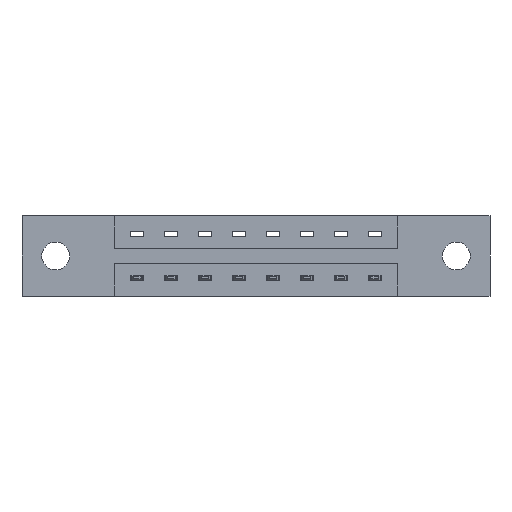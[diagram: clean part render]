
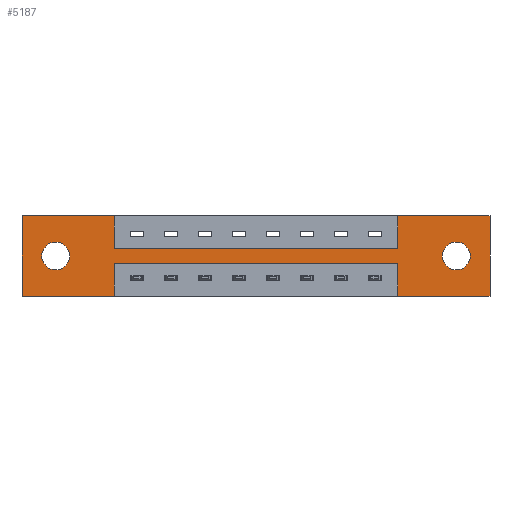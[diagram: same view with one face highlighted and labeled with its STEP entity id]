
A CAD part, front view. The second image highlights one B-rep face of the part: STEP entity #5187.
In plain terms, the highlighted planar face has unit normal (0, -1, 0).
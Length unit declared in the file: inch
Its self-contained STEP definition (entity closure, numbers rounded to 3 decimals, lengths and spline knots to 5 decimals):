
#52 = CARTESIAN_POINT ( 'NONE',  ( 1.729, 0., -0.37 ) ) ;
#64 = ORIENTED_EDGE ( 'NONE', *, *, #7880, .F. ) ;
#75 = CARTESIAN_POINT ( 'NONE',  ( 0.425, 0., -0.37 ) ) ;
#120 = CARTESIAN_POINT ( 'NONE',  ( 0., 0., 0. ) ) ;
#176 = CARTESIAN_POINT ( 'NONE',  ( 1.729, 0., 0. ) ) ;
#195 = LINE ( 'NONE', #4023, #8301 ) ;
#264 = CARTESIAN_POINT ( 'NONE',  ( 0., 0., 0. ) ) ;
#353 = ORIENTED_EDGE ( 'NONE', *, *, #9726, .F. ) ;
#450 = DIRECTION ( 'NONE',  ( 0., 1., 0. ) ) ;
#461 = VERTEX_POINT ( 'NONE', #4950 ) ;
#593 = VERTEX_POINT ( 'NONE', #9999 ) ;
#688 = LINE ( 'NONE', #8613, #2785 ) ;
#726 = EDGE_CURVE ( 'NONE', #593, #8300, #8420, .T. ) ;
#777 = EDGE_LOOP ( 'NONE', ( #1877, #1824 ) ) ;
#804 = CARTESIAN_POINT ( 'NONE',  ( 1.729, 0., -0.37 ) ) ;
#881 = LINE ( 'NONE', #1206, #3832 ) ;
#917 = CARTESIAN_POINT ( 'NONE',  ( 1.999, 0., -0.185 ) ) ;
#940 = VERTEX_POINT ( 'NONE', #6692 ) ;
#950 = DIRECTION ( 'NONE',  ( 0., 0., -1. ) ) ;
#1182 = EDGE_CURVE ( 'NONE', #461, #4940, #195, .T. ) ;
#1206 = CARTESIAN_POINT ( 'NONE',  ( 0., 0., 0. ) ) ;
#1278 = DIRECTION ( 'NONE',  ( 0., 1., 0. ) ) ;
#1452 = CIRCLE ( 'NONE', #3886, 0.064 ) ;
#1652 = LINE ( 'NONE', #5643, #7685 ) ;
#1708 = DIRECTION ( 'NONE',  ( 0., 1., 0. ) ) ;
#1778 = CIRCLE ( 'NONE', #5254, 0.064 ) ;
#1800 = EDGE_CURVE ( 'NONE', #6909, #2891, #7674, .T. ) ;
#1824 = ORIENTED_EDGE ( 'NONE', *, *, #1992, .T. ) ;
#1877 = ORIENTED_EDGE ( 'NONE', *, *, #9441, .T. ) ;
#1889 = DIRECTION ( 'NONE',  ( 0., 0., -1. ) ) ;
#1926 = VERTEX_POINT ( 'NONE', #7543 ) ;
#1992 = EDGE_CURVE ( 'NONE', #8514, #6498, #2105, .T. ) ;
#2105 = CIRCLE ( 'NONE', #4725, 0.064 ) ;
#2249 = DIRECTION ( 'NONE',  ( -1., 0., 0. ) ) ;
#2255 = CARTESIAN_POINT ( 'NONE',  ( 0., 0., -0.37 ) ) ;
#2265 = VECTOR ( 'NONE', #7362, 39.37008 ) ;
#2330 = EDGE_LOOP ( 'NONE', ( #5724, #7403, #7602, #4914, #9261, #9530, #353, #2766, #64, #7367, #5895, #9300 ) ) ;
#2389 = CARTESIAN_POINT ( 'NONE',  ( 0., 0., -0.37 ) ) ;
#2502 = EDGE_CURVE ( 'NONE', #2891, #1926, #881, .T. ) ;
#2766 = ORIENTED_EDGE ( 'NONE', *, *, #1182, .F. ) ;
#2785 = VECTOR ( 'NONE', #7009, 39.37008 ) ;
#2854 = DIRECTION ( 'NONE',  ( 0., 0., 1. ) ) ;
#2891 = VERTEX_POINT ( 'NONE', #120 ) ;
#3141 = CARTESIAN_POINT ( 'NONE',  ( 0.425, 0., -0.22 ) ) ;
#3403 = DIRECTION ( 'NONE',  ( 0., -1., 0. ) ) ;
#3424 = CARTESIAN_POINT ( 'NONE',  ( 0.155, 0., -0.121 ) ) ;
#3506 = PLANE ( 'NONE',  #7086 ) ;
#3513 = ORIENTED_EDGE ( 'NONE', *, *, #4875, .T. ) ;
#3809 = VERTEX_POINT ( 'NONE', #804 ) ;
#3832 = VECTOR ( 'NONE', #5127, 39.37008 ) ;
#3841 = EDGE_LOOP ( 'NONE', ( #3513, #7511 ) ) ;
#3884 = DIRECTION ( 'NONE',  ( 0., 0., -1. ) ) ;
#3886 = AXIS2_PLACEMENT_3D ( 'NONE', #6700, #1278, #5930 ) ;
#4023 = CARTESIAN_POINT ( 'NONE',  ( 0.425, 0., -0.15 ) ) ;
#4321 = CARTESIAN_POINT ( 'NONE',  ( 0., 0., -0.37 ) ) ;
#4501 = CIRCLE ( 'NONE', #9730, 0.064 ) ;
#4725 = AXIS2_PLACEMENT_3D ( 'NONE', #6296, #7839, #10087 ) ;
#4744 = DIRECTION ( 'NONE',  ( 0., 0., 1. ) ) ;
#4875 = EDGE_CURVE ( 'NONE', #940, #8865, #1452, .T. ) ;
#4914 = ORIENTED_EDGE ( 'NONE', *, *, #6810, .F. ) ;
#4940 = VERTEX_POINT ( 'NONE', #9097 ) ;
#4950 = CARTESIAN_POINT ( 'NONE',  ( 0.425, 0., -0.15 ) ) ;
#5127 = DIRECTION ( 'NONE',  ( 1., 0., 0. ) ) ;
#5187 = ADVANCED_FACE ( 'NONE', ( #5380, #8445, #6982 ), #3506, .T. ) ;
#5199 = LINE ( 'NONE', #2389, #8622 ) ;
#5254 = AXIS2_PLACEMENT_3D ( 'NONE', #7581, #450, #2854 ) ;
#5380 = FACE_BOUND ( 'NONE', #3841, .T. ) ;
#5643 = CARTESIAN_POINT ( 'NONE',  ( 1.729, 0., 0. ) ) ;
#5709 = VECTOR ( 'NONE', #6383, 39.37008 ) ;
#5724 = ORIENTED_EDGE ( 'NONE', *, *, #6390, .F. ) ;
#5735 = EDGE_CURVE ( 'NONE', #9885, #6605, #688, .T. ) ;
#5749 = VECTOR ( 'NONE', #8586, 39.37008 ) ;
#5837 = EDGE_CURVE ( 'NONE', #8865, #940, #4501, .T. ) ;
#5895 = ORIENTED_EDGE ( 'NONE', *, *, #1800, .F. ) ;
#5930 = DIRECTION ( 'NONE',  ( 0., 0., -1. ) ) ;
#6005 = DIRECTION ( 'NONE',  ( -1., 0., 0. ) ) ;
#6296 = CARTESIAN_POINT ( 'NONE',  ( 0.155, 0., -0.185 ) ) ;
#6314 = CARTESIAN_POINT ( 'NONE',  ( 0.425, 0., 0. ) ) ;
#6341 = CARTESIAN_POINT ( 'NONE',  ( 0.425, 0., -0.37 ) ) ;
#6383 = DIRECTION ( 'NONE',  ( 0., 0., 1. ) ) ;
#6390 = EDGE_CURVE ( 'NONE', #8300, #7465, #7914, .T. ) ;
#6497 = DIRECTION ( 'NONE',  ( 0., 0., 1. ) ) ;
#6498 = VERTEX_POINT ( 'NONE', #3424 ) ;
#6605 = VERTEX_POINT ( 'NONE', #8431 ) ;
#6692 = CARTESIAN_POINT ( 'NONE',  ( 1.999, 0., -0.121 ) ) ;
#6700 = CARTESIAN_POINT ( 'NONE',  ( 1.999, 0., -0.185 ) ) ;
#6810 = EDGE_CURVE ( 'NONE', #6605, #3809, #9123, .T. ) ;
#6909 = VERTEX_POINT ( 'NONE', #2255 ) ;
#6954 = CARTESIAN_POINT ( 'NONE',  ( 0.425, 0., -0.22 ) ) ;
#6982 = FACE_OUTER_BOUND ( 'NONE', #2330, .T. ) ;
#7009 = DIRECTION ( 'NONE',  ( 0., 0., -1. ) ) ;
#7086 = AXIS2_PLACEMENT_3D ( 'NONE', #4321, #3403, #7387 ) ;
#7155 = DIRECTION ( 'NONE',  ( 1., 0., 0. ) ) ;
#7172 = CARTESIAN_POINT ( 'NONE',  ( 1.999, 0., -0.249 ) ) ;
#7300 = CARTESIAN_POINT ( 'NONE',  ( 2.154, 0., 0. ) ) ;
#7342 = LINE ( 'NONE', #7999, #2265 ) ;
#7362 = DIRECTION ( 'NONE',  ( 1., 0., 0. ) ) ;
#7367 = ORIENTED_EDGE ( 'NONE', *, *, #2502, .F. ) ;
#7387 = DIRECTION ( 'NONE',  ( 0., 0., -1. ) ) ;
#7403 = ORIENTED_EDGE ( 'NONE', *, *, #726, .F. ) ;
#7465 = VERTEX_POINT ( 'NONE', #6341 ) ;
#7471 = EDGE_CURVE ( 'NONE', #3809, #593, #8389, .T. ) ;
#7511 = ORIENTED_EDGE ( 'NONE', *, *, #5837, .T. ) ;
#7543 = CARTESIAN_POINT ( 'NONE',  ( 0.425, 0., 0. ) ) ;
#7563 = VECTOR ( 'NONE', #4744, 39.37008 ) ;
#7577 = VECTOR ( 'NONE', #1889, 39.37008 ) ;
#7581 = CARTESIAN_POINT ( 'NONE',  ( 0.155, 0., -0.185 ) ) ;
#7602 = ORIENTED_EDGE ( 'NONE', *, *, #7471, .F. ) ;
#7674 = LINE ( 'NONE', #264, #7563 ) ;
#7685 = VECTOR ( 'NONE', #6497, 39.37008 ) ;
#7839 = DIRECTION ( 'NONE',  ( 0., 1., 0. ) ) ;
#7880 = EDGE_CURVE ( 'NONE', #1926, #461, #10070, .T. ) ;
#7914 = LINE ( 'NONE', #75, #7577 ) ;
#7999 = CARTESIAN_POINT ( 'NONE',  ( 0., 0., 0. ) ) ;
#8300 = VERTEX_POINT ( 'NONE', #6954 ) ;
#8301 = VECTOR ( 'NONE', #7155, 39.37008 ) ;
#8346 = EDGE_CURVE ( 'NONE', #7465, #6909, #5199, .T. ) ;
#8389 = LINE ( 'NONE', #52, #5709 ) ;
#8420 = LINE ( 'NONE', #3141, #5749 ) ;
#8431 = CARTESIAN_POINT ( 'NONE',  ( 2.154, 0., -0.37 ) ) ;
#8445 = FACE_BOUND ( 'NONE', #777, .T. ) ;
#8447 = CARTESIAN_POINT ( 'NONE',  ( 0., 0., -0.37 ) ) ;
#8494 = VERTEX_POINT ( 'NONE', #176 ) ;
#8514 = VERTEX_POINT ( 'NONE', #8767 ) ;
#8586 = DIRECTION ( 'NONE',  ( -1., 0., 0. ) ) ;
#8613 = CARTESIAN_POINT ( 'NONE',  ( 2.154, 0., 0. ) ) ;
#8622 = VECTOR ( 'NONE', #2249, 39.37008 ) ;
#8767 = CARTESIAN_POINT ( 'NONE',  ( 0.155, 0., -0.249 ) ) ;
#8865 = VERTEX_POINT ( 'NONE', #7172 ) ;
#8885 = VECTOR ( 'NONE', #3884, 39.37008 ) ;
#9022 = VECTOR ( 'NONE', #6005, 39.37008 ) ;
#9097 = CARTESIAN_POINT ( 'NONE',  ( 1.729, 0., -0.15 ) ) ;
#9123 = LINE ( 'NONE', #8447, #9022 ) ;
#9261 = ORIENTED_EDGE ( 'NONE', *, *, #5735, .F. ) ;
#9300 = ORIENTED_EDGE ( 'NONE', *, *, #8346, .F. ) ;
#9441 = EDGE_CURVE ( 'NONE', #6498, #8514, #1778, .T. ) ;
#9530 = ORIENTED_EDGE ( 'NONE', *, *, #9923, .F. ) ;
#9726 = EDGE_CURVE ( 'NONE', #4940, #8494, #1652, .T. ) ;
#9730 = AXIS2_PLACEMENT_3D ( 'NONE', #917, #1708, #950 ) ;
#9885 = VERTEX_POINT ( 'NONE', #7300 ) ;
#9923 = EDGE_CURVE ( 'NONE', #8494, #9885, #7342, .T. ) ;
#9999 = CARTESIAN_POINT ( 'NONE',  ( 1.729, 0., -0.22 ) ) ;
#10070 = LINE ( 'NONE', #6314, #8885 ) ;
#10087 = DIRECTION ( 'NONE',  ( 0., 0., 1. ) ) ;
